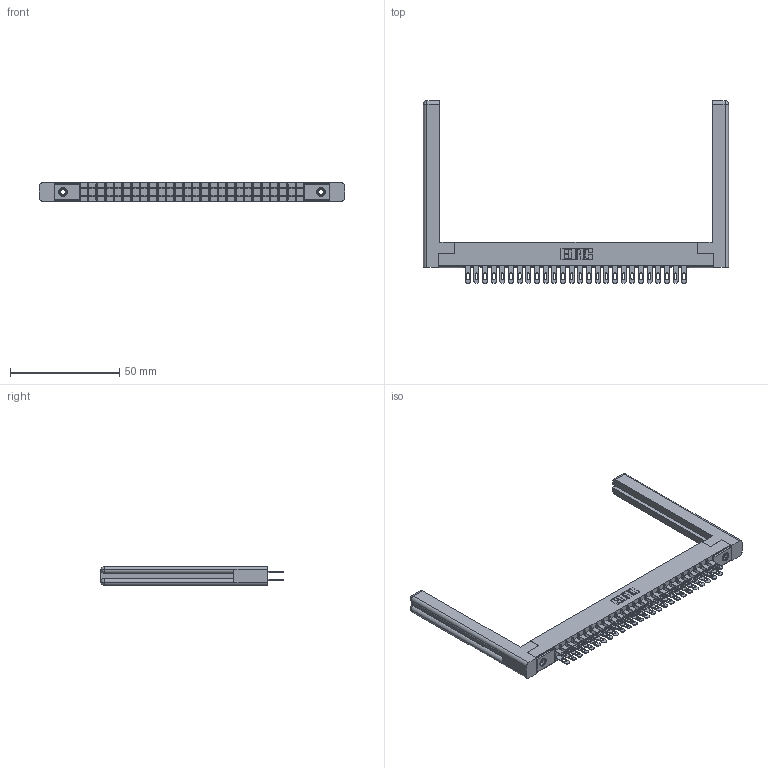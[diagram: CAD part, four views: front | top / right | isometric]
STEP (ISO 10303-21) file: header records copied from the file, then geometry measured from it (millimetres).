
FILE_DESCRIPTION (( 'STEP AP203' ), '1' );
FILE_NAME ('305-052-500-258.STEP', '2019-09-09T22:07:54', ( '' ), ( '' ), 'SwSTEP 2.0', 'SolidWorks 2016', '' );
FILE_SCHEMA (( 'CONFIG_CONTROL_DESIGN' ));
Length unit declared in the file: inch
Products named in the file (5): 307-220-058; 345-250-001_345-250-001-102; 305-052-500-258; 305-290-001_500; 305 Part_.156 Dia
Assembly tree (57 placements, depth 2):
  305-052-500-258
    305 Part_.156 Dia
    305-290-001_500  x52
    345-250-001_345-250-001-102  x2
    307-220-058  x2
Bounding box: 139.65 x 83.49 x 8.71 mm (x, y, z)
Volume: 16632.1 mm3; surface area: 23036 mm2
Topology: 57 solids, 57 shells, 2858 faces, 8132 edges, 5268 vertices
Faces by surface type: plane 1608, cylinder 1122, sphere 104, cone 12, torus 12
Entity records: 32754 total; most frequent: CARTESIAN_POINT 5435, ORIENTED_EDGE 5334, DIRECTION 5235, EDGE_CURVE 2667, VECTOR 2127, LINE 2127, VERTEX_POINT 1700, AXIS2_PLACEMENT_3D 1554
